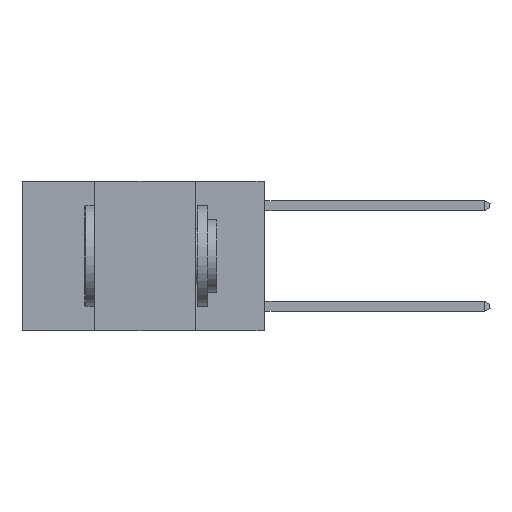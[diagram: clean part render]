
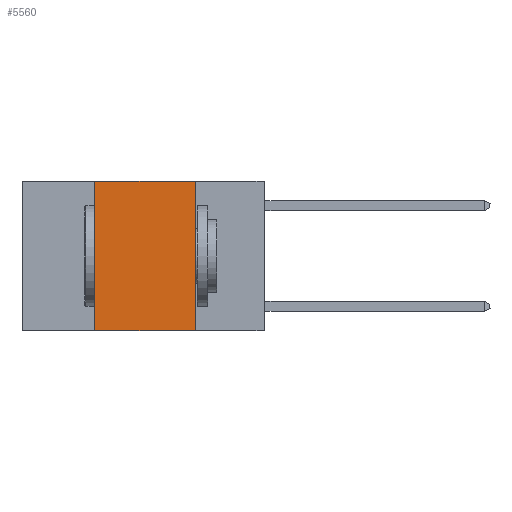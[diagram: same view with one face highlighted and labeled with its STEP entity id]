
A CAD part, left-side view. The second image highlights one B-rep face of the part: STEP entity #5560.
In plain terms, the highlighted planar face has unit normal (-1, 0, 0).
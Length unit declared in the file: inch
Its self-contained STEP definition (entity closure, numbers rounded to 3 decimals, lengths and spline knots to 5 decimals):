
#603 = DIRECTION ( 'NONE',  ( 0., 0., 1. ) ) ;
#606 = LINE ( 'NONE', #14110, #12240 ) ;
#644 = CARTESIAN_POINT ( 'NONE',  ( 0., 0.6, -0.37 ) ) ;
#775 = CARTESIAN_POINT ( 'NONE',  ( 0., 0.6, 0. ) ) ;
#1209 = ORIENTED_EDGE ( 'NONE', *, *, #15519, .F. ) ;
#1697 = CARTESIAN_POINT ( 'NONE',  ( 0., 0.6, 0. ) ) ;
#1782 = DIRECTION ( 'NONE',  ( 0., -1., 0. ) ) ;
#1854 = PLANE ( 'NONE',  #7381 ) ;
#1866 = ORIENTED_EDGE ( 'NONE', *, *, #10903, .T. ) ;
#2065 = ORIENTED_EDGE ( 'NONE', *, *, #14869, .F. ) ;
#2932 = VECTOR ( 'NONE', #603, 39.37008 ) ;
#4344 = LINE ( 'NONE', #644, #14166 ) ;
#5179 = CARTESIAN_POINT ( 'NONE',  ( 0., 0.17, 0. ) ) ;
#5560 = ADVANCED_FACE ( 'NONE', ( #9264 ), #1854, .F. ) ;
#6274 = CARTESIAN_POINT ( 'NONE',  ( 0., 0.42, -0.37 ) ) ;
#7381 = AXIS2_PLACEMENT_3D ( 'NONE', #1697, #13747, #8065 ) ;
#7940 = CARTESIAN_POINT ( 'NONE',  ( 0., 0.42, 0. ) ) ;
#7944 = DIRECTION ( 'NONE',  ( 0., 0., -1. ) ) ;
#8007 = VERTEX_POINT ( 'NONE', #11156 ) ;
#8065 = DIRECTION ( 'NONE',  ( 0., 0., -1. ) ) ;
#8222 = VECTOR ( 'NONE', #15219, 39.37008 ) ;
#9148 = LINE ( 'NONE', #7940, #2932 ) ;
#9231 = LINE ( 'NONE', #775, #8222 ) ;
#9264 = FACE_OUTER_BOUND ( 'NONE', #9979, .T. ) ;
#9979 = EDGE_LOOP ( 'NONE', ( #2065, #14131, #1209, #1866 ) ) ;
#10903 = EDGE_CURVE ( 'NONE', #12567, #11336, #4344, .T. ) ;
#11156 = CARTESIAN_POINT ( 'NONE',  ( 0., 0.42, 0. ) ) ;
#11336 = VERTEX_POINT ( 'NONE', #12471 ) ;
#12240 = VECTOR ( 'NONE', #7944, 39.37008 ) ;
#12471 = CARTESIAN_POINT ( 'NONE',  ( 0., 0.17, -0.37 ) ) ;
#12567 = VERTEX_POINT ( 'NONE', #6274 ) ;
#13621 = VERTEX_POINT ( 'NONE', #5179 ) ;
#13747 = DIRECTION ( 'NONE',  ( 1., 0., 0. ) ) ;
#14110 = CARTESIAN_POINT ( 'NONE',  ( 0., 0.17, 0. ) ) ;
#14131 = ORIENTED_EDGE ( 'NONE', *, *, #14822, .F. ) ;
#14166 = VECTOR ( 'NONE', #1782, 39.37008 ) ;
#14822 = EDGE_CURVE ( 'NONE', #8007, #13621, #9231, .T. ) ;
#14869 = EDGE_CURVE ( 'NONE', #13621, #11336, #606, .T. ) ;
#15219 = DIRECTION ( 'NONE',  ( 0., -1., 0. ) ) ;
#15519 = EDGE_CURVE ( 'NONE', #12567, #8007, #9148, .T. ) ;
